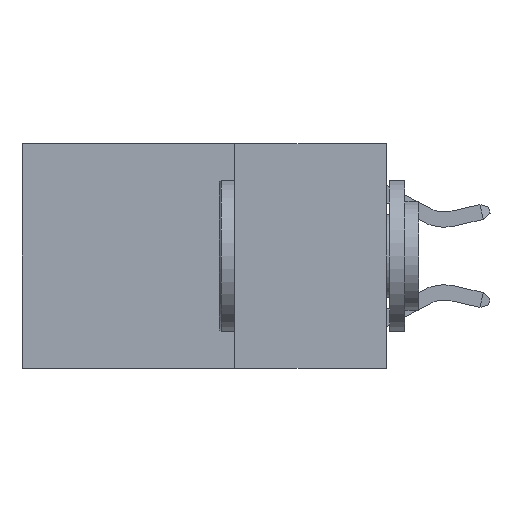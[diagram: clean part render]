
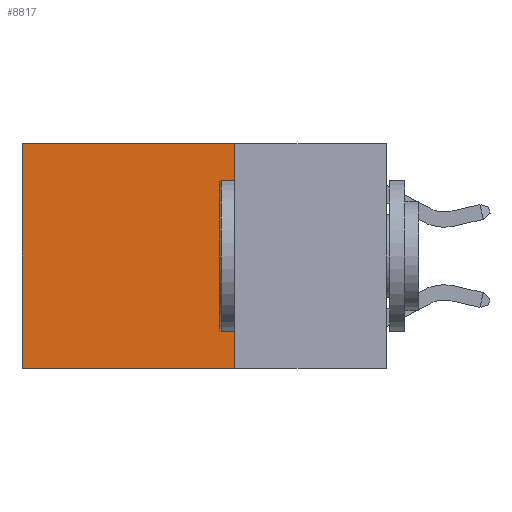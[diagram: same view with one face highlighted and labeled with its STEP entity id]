
A CAD part, left-side view. The second image highlights one B-rep face of the part: STEP entity #8817.
In plain terms, the highlighted planar face has unit normal (-1, 0, 0).
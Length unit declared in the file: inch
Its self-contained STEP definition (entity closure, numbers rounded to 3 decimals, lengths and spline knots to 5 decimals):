
#17 = CARTESIAN_POINT ( 'NONE',  ( 0.2625, 0.25, 0. ) ) ;
#361 = DIRECTION ( 'NONE',  ( 0., 0., -1. ) ) ;
#502 = VECTOR ( 'NONE', #7859, 39.37008 ) ;
#550 = DIRECTION ( 'NONE',  ( 1., 0., 0. ) ) ;
#553 = VECTOR ( 'NONE', #3380, 39.37008 ) ;
#1046 = VERTEX_POINT ( 'NONE', #9743 ) ;
#1995 = ORIENTED_EDGE ( 'NONE', *, *, #3443, .T. ) ;
#2524 = DIRECTION ( 'NONE',  ( 0., 1., 0. ) ) ;
#2830 = LINE ( 'NONE', #9255, #553 ) ;
#3380 = DIRECTION ( 'NONE',  ( 0., 1., 0. ) ) ;
#3422 = CARTESIAN_POINT ( 'NONE',  ( 0.2625, 0.25, -0.37 ) ) ;
#3443 = EDGE_CURVE ( 'NONE', #12846, #1046, #2830, .T. ) ;
#3528 = DIRECTION ( 'NONE',  ( 0., 0., -1. ) ) ;
#3866 = EDGE_LOOP ( 'NONE', ( #15839, #18003, #18483, #1995 ) ) ;
#3998 = CARTESIAN_POINT ( 'NONE',  ( 0.2625, 0.25, -0.37 ) ) ;
#4388 = LINE ( 'NONE', #10715, #502 ) ;
#4858 = PLANE ( 'NONE',  #16205 ) ;
#5070 = EDGE_CURVE ( 'NONE', #12846, #5832, #4388, .T. ) ;
#5832 = VERTEX_POINT ( 'NONE', #3422 ) ;
#7435 = VERTEX_POINT ( 'NONE', #11950 ) ;
#7702 = LINE ( 'NONE', #3998, #9765 ) ;
#7859 = DIRECTION ( 'NONE',  ( 0., 0., -1. ) ) ;
#7975 = EDGE_CURVE ( 'NONE', #1046, #7435, #13007, .T. ) ;
#8817 = ADVANCED_FACE ( 'NONE', ( #13435 ), #4858, .F. ) ;
#9255 = CARTESIAN_POINT ( 'NONE',  ( 0.2625, 0.25, 0. ) ) ;
#9743 = CARTESIAN_POINT ( 'NONE',  ( 0.2625, 0.6, 0. ) ) ;
#9765 = VECTOR ( 'NONE', #2524, 39.37008 ) ;
#9814 = EDGE_CURVE ( 'NONE', #5832, #7435, #7702, .T. ) ;
#10715 = CARTESIAN_POINT ( 'NONE',  ( 0.2625, 0.25, 0. ) ) ;
#11950 = CARTESIAN_POINT ( 'NONE',  ( 0.2625, 0.6, -0.37 ) ) ;
#12846 = VERTEX_POINT ( 'NONE', #17 ) ;
#13007 = LINE ( 'NONE', #15236, #18062 ) ;
#13435 = FACE_OUTER_BOUND ( 'NONE', #3866, .T. ) ;
#15236 = CARTESIAN_POINT ( 'NONE',  ( 0.2625, 0.6, 0. ) ) ;
#15839 = ORIENTED_EDGE ( 'NONE', *, *, #7975, .T. ) ;
#16205 = AXIS2_PLACEMENT_3D ( 'NONE', #17929, #550, #361 ) ;
#17929 = CARTESIAN_POINT ( 'NONE',  ( 0.2625, 0.25, 0. ) ) ;
#18003 = ORIENTED_EDGE ( 'NONE', *, *, #9814, .F. ) ;
#18062 = VECTOR ( 'NONE', #3528, 39.37008 ) ;
#18483 = ORIENTED_EDGE ( 'NONE', *, *, #5070, .F. ) ;
